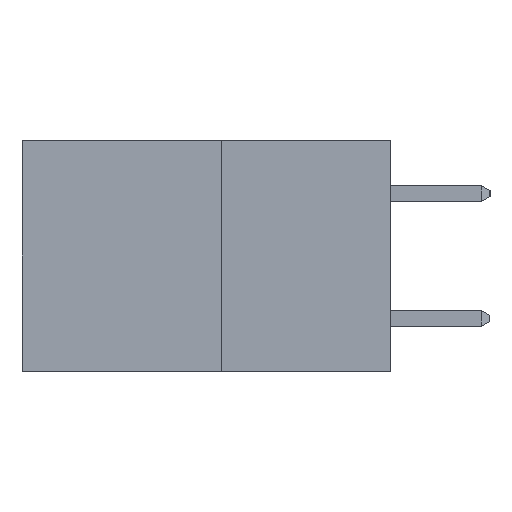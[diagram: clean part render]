
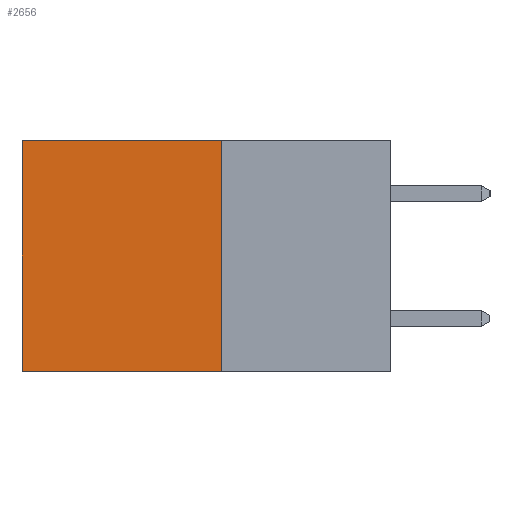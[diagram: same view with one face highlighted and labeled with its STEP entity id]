
A CAD part, left-side view. The second image highlights one B-rep face of the part: STEP entity #2656.
In plain terms, the highlighted planar face has unit normal (-1, 0, 0).
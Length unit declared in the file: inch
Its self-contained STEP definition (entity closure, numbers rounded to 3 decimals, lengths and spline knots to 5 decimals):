
#230 = EDGE_CURVE ( 'NONE', #3798, #2826, #4895, .T. ) ;
#433 = VECTOR ( 'NONE', #2339, 39.37008 ) ;
#437 = EDGE_LOOP ( 'NONE', ( #1118, #1316, #7078, #3757 ) ) ;
#602 = VERTEX_POINT ( 'NONE', #4612 ) ;
#1118 = ORIENTED_EDGE ( 'NONE', *, *, #5933, .T. ) ;
#1316 = ORIENTED_EDGE ( 'NONE', *, *, #4366, .F. ) ;
#1449 = EDGE_CURVE ( 'NONE', #3798, #602, #1769, .T. ) ;
#1742 = PLANE ( 'NONE',  #6388 ) ;
#1756 = DIRECTION ( 'NONE',  ( 0., 1., 0. ) ) ;
#1765 = DIRECTION ( 'NONE',  ( 0., 0., -1. ) ) ;
#1769 = LINE ( 'NONE', #7819, #10132 ) ;
#1860 = CARTESIAN_POINT ( 'NONE',  ( 0.277, 0.27, 0. ) ) ;
#2119 = DIRECTION ( 'NONE',  ( 1., 0., 0. ) ) ;
#2221 = CARTESIAN_POINT ( 'NONE',  ( 0.277, 0.27, 0. ) ) ;
#2339 = DIRECTION ( 'NONE',  ( 0., 1., 0. ) ) ;
#2656 = ADVANCED_FACE ( 'NONE', ( #6663 ), #1742, .F. ) ;
#2826 = VERTEX_POINT ( 'NONE', #5618 ) ;
#3014 = CARTESIAN_POINT ( 'NONE',  ( 0.277, 0.27, -0.37 ) ) ;
#3322 = CARTESIAN_POINT ( 'NONE',  ( 0.277, 0.59, -0.37 ) ) ;
#3757 = ORIENTED_EDGE ( 'NONE', *, *, #230, .T. ) ;
#3798 = VERTEX_POINT ( 'NONE', #1860 ) ;
#3883 = CARTESIAN_POINT ( 'NONE',  ( 0.277, 0.27, -0.37 ) ) ;
#3901 = VECTOR ( 'NONE', #1756, 39.37008 ) ;
#4366 = EDGE_CURVE ( 'NONE', #602, #8818, #8186, .T. ) ;
#4558 = DIRECTION ( 'NONE',  ( 0., 0., -1. ) ) ;
#4612 = CARTESIAN_POINT ( 'NONE',  ( 0.277, 0.27, -0.37 ) ) ;
#4895 = LINE ( 'NONE', #2221, #433 ) ;
#5618 = CARTESIAN_POINT ( 'NONE',  ( 0.277, 0.59, 0. ) ) ;
#5933 = EDGE_CURVE ( 'NONE', #2826, #8818, #8276, .T. ) ;
#6388 = AXIS2_PLACEMENT_3D ( 'NONE', #3883, #2119, #1765 ) ;
#6663 = FACE_OUTER_BOUND ( 'NONE', #437, .T. ) ;
#7078 = ORIENTED_EDGE ( 'NONE', *, *, #1449, .F. ) ;
#7370 = DIRECTION ( 'NONE',  ( 0., 0., -1. ) ) ;
#7727 = CARTESIAN_POINT ( 'NONE',  ( 0.277, 0.59, -0.37 ) ) ;
#7819 = CARTESIAN_POINT ( 'NONE',  ( 0.277, 0.27, -0.37 ) ) ;
#8186 = LINE ( 'NONE', #3014, #3901 ) ;
#8276 = LINE ( 'NONE', #7727, #10344 ) ;
#8818 = VERTEX_POINT ( 'NONE', #3322 ) ;
#10132 = VECTOR ( 'NONE', #4558, 39.37008 ) ;
#10344 = VECTOR ( 'NONE', #7370, 39.37008 ) ;
